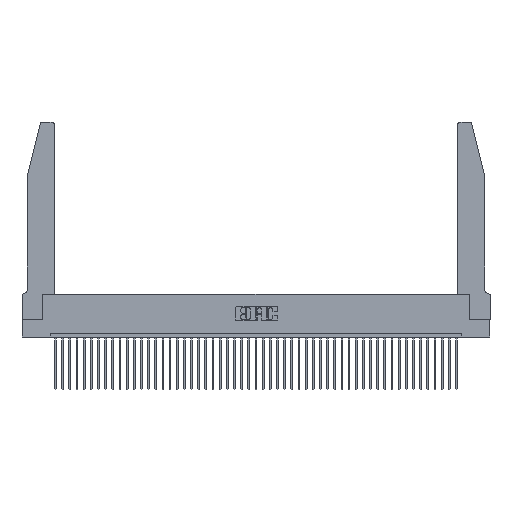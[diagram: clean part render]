
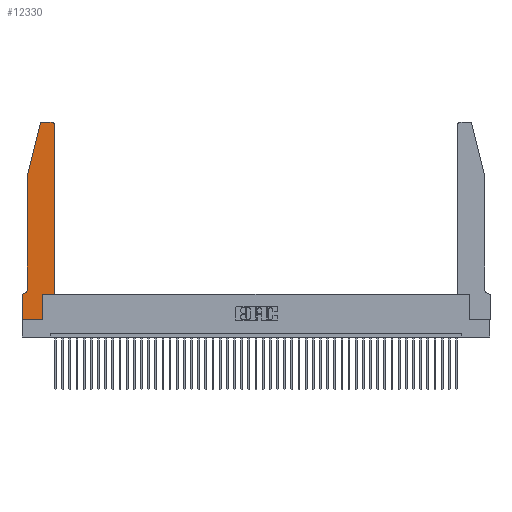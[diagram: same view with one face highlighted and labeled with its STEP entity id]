
A CAD part, top view. The second image highlights one B-rep face of the part: STEP entity #12330.
In plain terms, the highlighted planar face has unit normal (0, 0, 1).
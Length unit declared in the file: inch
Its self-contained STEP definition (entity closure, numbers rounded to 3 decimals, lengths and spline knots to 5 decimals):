
#290 = LINE ( 'NONE', #24102, #5240 ) ;
#398 = CARTESIAN_POINT ( 'NONE',  ( 0., 0.35, 0.37 ) ) ;
#942 = EDGE_CURVE ( 'NONE', #37867, #38849, #3037, .T. ) ;
#1266 = CARTESIAN_POINT ( 'NONE',  ( 0.284, 2.75, 0.37 ) ) ;
#1304 = ORIENTED_EDGE ( 'NONE', *, *, #34521, .T. ) ;
#1382 = VECTOR ( 'NONE', #16252, 39.37008 ) ;
#1537 = DIRECTION ( 'NONE',  ( 0., 0., 1. ) ) ;
#2316 = CARTESIAN_POINT ( 'NONE',  ( 0.0755, 0.35, 0.37 ) ) ;
#2719 = CIRCLE ( 'NONE', #19208, 0.03 ) ;
#3037 = LINE ( 'NONE', #26623, #1382 ) ;
#3342 = CARTESIAN_POINT ( 'NONE',  ( 0., 0.35, 0.37 ) ) ;
#4316 = CARTESIAN_POINT ( 'NONE',  ( 0.4505, 0.35, 0.37 ) ) ;
#5240 = VECTOR ( 'NONE', #13026, 39.37008 ) ;
#5355 = ORIENTED_EDGE ( 'NONE', *, *, #32789, .T. ) ;
#5375 = DIRECTION ( 'NONE',  ( -1., 0., 0. ) ) ;
#5509 = DIRECTION ( 'NONE',  ( 1., 0., 0. ) ) ;
#5784 = EDGE_CURVE ( 'NONE', #26192, #18451, #6946, .T. ) ;
#5938 = CARTESIAN_POINT ( 'NONE',  ( 0.0755, 2., 0.37 ) ) ;
#6423 = EDGE_CURVE ( 'NONE', #12917, #26192, #15182, .T. ) ;
#6815 = AXIS2_PLACEMENT_3D ( 'NONE', #18870, #8643, #5375 ) ;
#6880 = DIRECTION ( 'NONE',  ( 1., 0., 0. ) ) ;
#6946 = LINE ( 'NONE', #12739, #45027 ) ;
#7007 = ORIENTED_EDGE ( 'NONE', *, *, #11145, .T. ) ;
#7054 = VERTEX_POINT ( 'NONE', #30139 ) ;
#7859 = ORIENTED_EDGE ( 'NONE', *, *, #32021, .T. ) ;
#8291 = DIRECTION ( 'NONE',  ( 0., 1., 0. ) ) ;
#8643 = DIRECTION ( 'NONE',  ( 0., 0., -1. ) ) ;
#8777 = CARTESIAN_POINT ( 'NONE',  ( 0.284, 2.72, 0.37 ) ) ;
#9637 = ORIENTED_EDGE ( 'NONE', *, *, #5784, .T. ) ;
#10729 = CIRCLE ( 'NONE', #30650, 0.03 ) ;
#11145 = EDGE_CURVE ( 'NONE', #40231, #42519, #10729, .T. ) ;
#11156 = FACE_OUTER_BOUND ( 'NONE', #17606, .T. ) ;
#11336 = CARTESIAN_POINT ( 'NONE',  ( 0.2865, 0.35, 0.37 ) ) ;
#11937 = LINE ( 'NONE', #30362, #18012 ) ;
#12330 = ADVANCED_FACE ( 'NONE', ( #11156 ), #24455, .T. ) ;
#12739 = CARTESIAN_POINT ( 'NONE',  ( 0.4505, 0.35, 0.37 ) ) ;
#12917 = VERTEX_POINT ( 'NONE', #11336 ) ;
#13026 = DIRECTION ( 'NONE',  ( 1., 0., 0. ) ) ;
#15182 = LINE ( 'NONE', #22775, #26807 ) ;
#15371 = DIRECTION ( 'NONE',  ( 1., 0., 0. ) ) ;
#15703 = CARTESIAN_POINT ( 'NONE',  ( 0.0755, 0.42, 0.37 ) ) ;
#16127 = LINE ( 'NONE', #2316, #44209 ) ;
#16252 = DIRECTION ( 'NONE',  ( 0., -1., 0. ) ) ;
#16668 = CIRCLE ( 'NONE', #6815, 0.07 ) ;
#17606 = EDGE_LOOP ( 'NONE', ( #41761, #7007, #7859, #39026, #30569, #1304, #37186, #5355, #22411, #40627, #9637, #18124 ) ) ;
#18012 = VECTOR ( 'NONE', #27291, 39.37008 ) ;
#18124 = ORIENTED_EDGE ( 'NONE', *, *, #23449, .T. ) ;
#18193 = DIRECTION ( 'NONE',  ( 1., 0., 0. ) ) ;
#18271 = CARTESIAN_POINT ( 'NONE',  ( 0.4505, 2.72, 0.37 ) ) ;
#18451 = VERTEX_POINT ( 'NONE', #18271 ) ;
#18561 = AXIS2_PLACEMENT_3D ( 'NONE', #3342, #28055, #6880 ) ;
#18870 = CARTESIAN_POINT ( 'NONE',  ( 0.0055, 0.42, 0.37 ) ) ;
#19208 = AXIS2_PLACEMENT_3D ( 'NONE', #24960, #25132, #18193 ) ;
#20650 = DIRECTION ( 'NONE',  ( 0., 1., 0. ) ) ;
#21997 = CARTESIAN_POINT ( 'NONE',  ( 0.4205, 2.75, 0.37 ) ) ;
#22411 = ORIENTED_EDGE ( 'NONE', *, *, #28571, .T. ) ;
#22613 = VECTOR ( 'NONE', #25524, 39.37008 ) ;
#22775 = CARTESIAN_POINT ( 'NONE',  ( 0.4505, 0.35, 0.37 ) ) ;
#23449 = EDGE_CURVE ( 'NONE', #18451, #26520, #2719, .T. ) ;
#24102 = CARTESIAN_POINT ( 'NONE',  ( 0., 0., 0.37 ) ) ;
#24455 = PLANE ( 'NONE',  #18561 ) ;
#24960 = CARTESIAN_POINT ( 'NONE',  ( 0.4205, 2.72, 0.37 ) ) ;
#25132 = DIRECTION ( 'NONE',  ( 0., 0., 1. ) ) ;
#25524 = DIRECTION ( 'NONE',  ( 0., -1., 0. ) ) ;
#25915 = VECTOR ( 'NONE', #40385, 39.37008 ) ;
#25926 = LINE ( 'NONE', #29080, #22613 ) ;
#26057 = LINE ( 'NONE', #36189, #30501 ) ;
#26192 = VERTEX_POINT ( 'NONE', #4316 ) ;
#26520 = VERTEX_POINT ( 'NONE', #21997 ) ;
#26623 = CARTESIAN_POINT ( 'NONE',  ( 0.0755, 2., 0.37 ) ) ;
#26635 = CARTESIAN_POINT ( 'NONE',  ( 0.25487, 2.72718, 0.37 ) ) ;
#26807 = VECTOR ( 'NONE', #15371, 39.37008 ) ;
#27002 = DIRECTION ( 'NONE',  ( -1., 0., 0. ) ) ;
#27291 = DIRECTION ( 'NONE',  ( -0.239, -0.971, 0. ) ) ;
#28055 = DIRECTION ( 'NONE',  ( 0., 0., 1. ) ) ;
#28571 = EDGE_CURVE ( 'NONE', #43201, #12917, #26057, .T. ) ;
#29069 = VERTEX_POINT ( 'NONE', #398 ) ;
#29080 = CARTESIAN_POINT ( 'NONE',  ( 0., 0., 0.37 ) ) ;
#29553 = CARTESIAN_POINT ( 'NONE',  ( 0., 0., 0.37 ) ) ;
#30139 = CARTESIAN_POINT ( 'NONE',  ( 0.0055, 0.35, 0.37 ) ) ;
#30362 = CARTESIAN_POINT ( 'NONE',  ( 0.0755, 2., 0.37 ) ) ;
#30501 = VECTOR ( 'NONE', #8291, 39.37008 ) ;
#30569 = ORIENTED_EDGE ( 'NONE', *, *, #34394, .T. ) ;
#30595 = EDGE_CURVE ( 'NONE', #29069, #30783, #25926, .T. ) ;
#30650 = AXIS2_PLACEMENT_3D ( 'NONE', #8777, #1537, #5509 ) ;
#30783 = VERTEX_POINT ( 'NONE', #29553 ) ;
#32021 = EDGE_CURVE ( 'NONE', #42519, #37867, #11937, .T. ) ;
#32789 = EDGE_CURVE ( 'NONE', #30783, #43201, #290, .T. ) ;
#32871 = CARTESIAN_POINT ( 'NONE',  ( 0.2865, 0., 0.37 ) ) ;
#33505 = CARTESIAN_POINT ( 'NONE',  ( 0.2605, 2.75, 0.37 ) ) ;
#34394 = EDGE_CURVE ( 'NONE', #38849, #7054, #16668, .T. ) ;
#34521 = EDGE_CURVE ( 'NONE', #7054, #29069, #16127, .T. ) ;
#35265 = LINE ( 'NONE', #33505, #25915 ) ;
#35778 = EDGE_CURVE ( 'NONE', #26520, #40231, #35265, .T. ) ;
#36189 = CARTESIAN_POINT ( 'NONE',  ( 0.2865, 0.35, 0.37 ) ) ;
#37186 = ORIENTED_EDGE ( 'NONE', *, *, #30595, .T. ) ;
#37867 = VERTEX_POINT ( 'NONE', #5938 ) ;
#38849 = VERTEX_POINT ( 'NONE', #15703 ) ;
#39026 = ORIENTED_EDGE ( 'NONE', *, *, #942, .T. ) ;
#40231 = VERTEX_POINT ( 'NONE', #1266 ) ;
#40385 = DIRECTION ( 'NONE',  ( -1., 0., 0. ) ) ;
#40627 = ORIENTED_EDGE ( 'NONE', *, *, #6423, .T. ) ;
#41761 = ORIENTED_EDGE ( 'NONE', *, *, #35778, .T. ) ;
#42519 = VERTEX_POINT ( 'NONE', #26635 ) ;
#43201 = VERTEX_POINT ( 'NONE', #32871 ) ;
#44209 = VECTOR ( 'NONE', #27002, 39.37008 ) ;
#45027 = VECTOR ( 'NONE', #20650, 39.37008 ) ;
